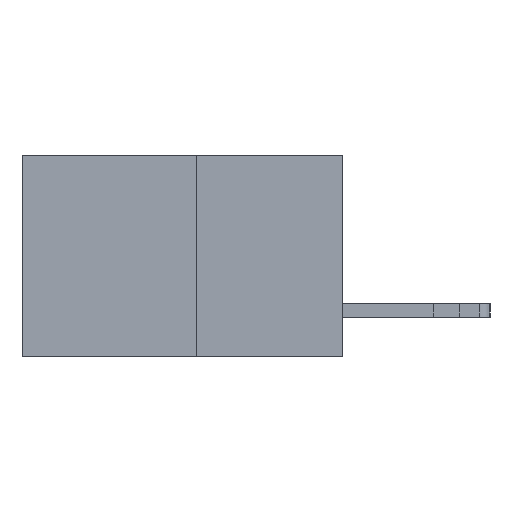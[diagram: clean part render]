
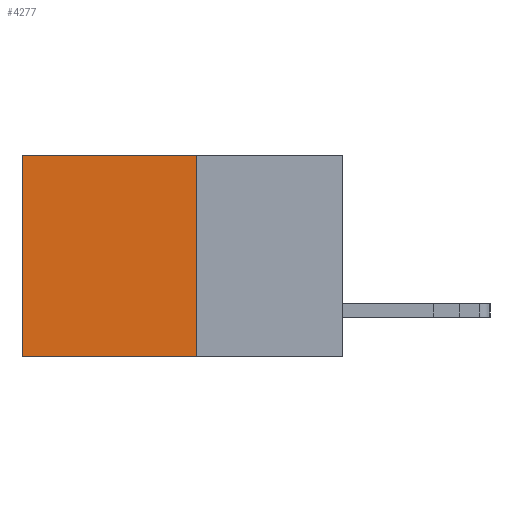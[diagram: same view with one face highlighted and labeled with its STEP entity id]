
A CAD part, left-side view. The second image highlights one B-rep face of the part: STEP entity #4277.
In plain terms, the highlighted planar face has unit normal (-1, 0, 0).
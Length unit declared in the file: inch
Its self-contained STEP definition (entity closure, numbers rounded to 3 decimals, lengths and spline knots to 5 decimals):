
#147 = VECTOR ( 'NONE', #10206, 39.37008 ) ;
#589 = DIRECTION ( 'NONE',  ( 0., 0., -1. ) ) ;
#600 = LINE ( 'NONE', #11561, #11264 ) ;
#825 = EDGE_LOOP ( 'NONE', ( #4423, #2664, #12344, #6474 ) ) ;
#993 = VERTEX_POINT ( 'NONE', #12464 ) ;
#2255 = FACE_OUTER_BOUND ( 'NONE', #825, .T. ) ;
#2427 = AXIS2_PLACEMENT_3D ( 'NONE', #5096, #3068, #589 ) ;
#2664 = ORIENTED_EDGE ( 'NONE', *, *, #8328, .F. ) ;
#3068 = DIRECTION ( 'NONE',  ( 1., 0., 0. ) ) ;
#3187 = CARTESIAN_POINT ( 'NONE',  ( 0.277, 0.59, 0. ) ) ;
#3243 = PLANE ( 'NONE',  #2427 ) ;
#3940 = LINE ( 'NONE', #8367, #11167 ) ;
#4187 = EDGE_CURVE ( 'NONE', #12258, #6318, #5301, .T. ) ;
#4277 = ADVANCED_FACE ( 'NONE', ( #2255 ), #3243, .F. ) ;
#4423 = ORIENTED_EDGE ( 'NONE', *, *, #12816, .T. ) ;
#4689 = DIRECTION ( 'NONE',  ( 0., 1., 0. ) ) ;
#4942 = CARTESIAN_POINT ( 'NONE',  ( 0.277, 0.27, -0.37 ) ) ;
#5096 = CARTESIAN_POINT ( 'NONE',  ( 0.277, 0.27, -0.37 ) ) ;
#5301 = LINE ( 'NONE', #4942, #10174 ) ;
#6318 = VERTEX_POINT ( 'NONE', #10902 ) ;
#6452 = DIRECTION ( 'NONE',  ( 0., 0., -1. ) ) ;
#6474 = ORIENTED_EDGE ( 'NONE', *, *, #11291, .T. ) ;
#7225 = VERTEX_POINT ( 'NONE', #3187 ) ;
#7632 = DIRECTION ( 'NONE',  ( 0., 0., -1. ) ) ;
#8328 = EDGE_CURVE ( 'NONE', #6318, #993, #10873, .T. ) ;
#8367 = CARTESIAN_POINT ( 'NONE',  ( 0.277, 0.59, -0.37 ) ) ;
#10174 = VECTOR ( 'NONE', #7632, 39.37008 ) ;
#10206 = DIRECTION ( 'NONE',  ( 0., 1., 0. ) ) ;
#10414 = CARTESIAN_POINT ( 'NONE',  ( 0.277, 0.27, 0. ) ) ;
#10873 = LINE ( 'NONE', #12113, #147 ) ;
#10902 = CARTESIAN_POINT ( 'NONE',  ( 0.277, 0.27, -0.37 ) ) ;
#11167 = VECTOR ( 'NONE', #6452, 39.37008 ) ;
#11264 = VECTOR ( 'NONE', #4689, 39.37008 ) ;
#11291 = EDGE_CURVE ( 'NONE', #12258, #7225, #600, .T. ) ;
#11561 = CARTESIAN_POINT ( 'NONE',  ( 0.277, 0.27, 0. ) ) ;
#12113 = CARTESIAN_POINT ( 'NONE',  ( 0.277, 0.27, -0.37 ) ) ;
#12258 = VERTEX_POINT ( 'NONE', #10414 ) ;
#12344 = ORIENTED_EDGE ( 'NONE', *, *, #4187, .F. ) ;
#12464 = CARTESIAN_POINT ( 'NONE',  ( 0.277, 0.59, -0.37 ) ) ;
#12816 = EDGE_CURVE ( 'NONE', #7225, #993, #3940, .T. ) ;
